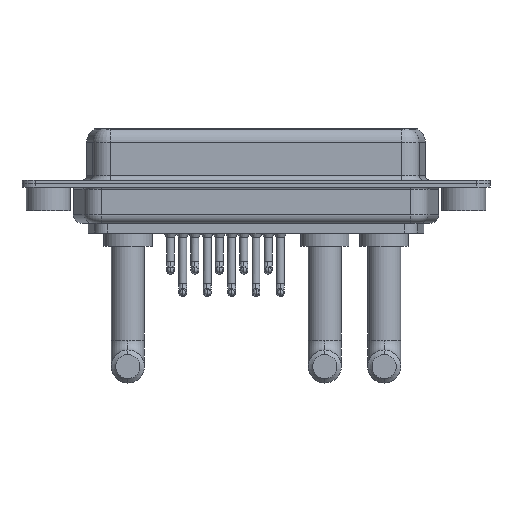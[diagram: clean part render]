
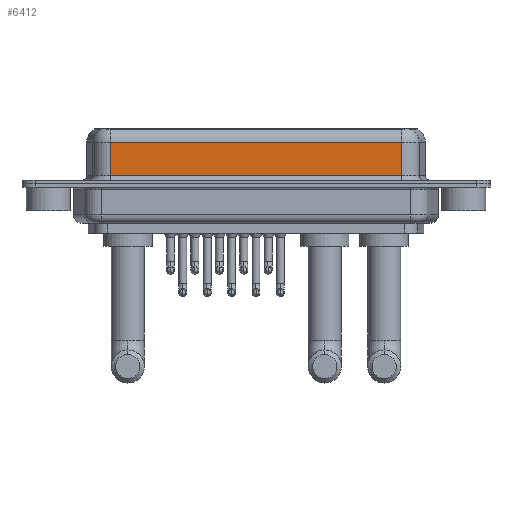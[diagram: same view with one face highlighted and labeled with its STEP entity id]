
A CAD part, front view. The second image highlights one B-rep face of the part: STEP entity #6412.
In plain terms, the highlighted planar face has unit normal (0, -1, 0).
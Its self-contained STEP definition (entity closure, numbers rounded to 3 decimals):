
#167 = CARTESIAN_POINT ( 'NONE',  ( 7.013, -3.95, 0.9 ) ) ;
#1399 = CARTESIAN_POINT ( 'NONE',  ( 40.037, -3.95, 4.65 ) ) ;
#1458 = CARTESIAN_POINT ( 'NONE',  ( 40.037, -3.95, 0.9 ) ) ;
#1975 = AXIS2_PLACEMENT_3D ( 'NONE', #12517, #11176, #11276 ) ;
#2975 = VECTOR ( 'NONE', #13521, 1000. ) ;
#3056 = VECTOR ( 'NONE', #12246, 1000. ) ;
#4353 = CARTESIAN_POINT ( 'NONE',  ( 7.013, -3.95, 6.4 ) ) ;
#5271 = VECTOR ( 'NONE', #11864, 1000. ) ;
#5887 = LINE ( 'NONE', #4353, #5271 ) ;
#6412 = ADVANCED_FACE ( 'NONE', ( #6461 ), #15302, .F. ) ;
#6461 = FACE_OUTER_BOUND ( 'NONE', #9203, .T. ) ;
#7152 = VERTEX_POINT ( 'NONE', #1399 ) ;
#7917 = ORIENTED_EDGE ( 'NONE', *, *, #9746, .T. ) ;
#8145 = LINE ( 'NONE', #16818, #17758 ) ;
#8759 = ORIENTED_EDGE ( 'NONE', *, *, #16639, .T. ) ;
#8780 = VERTEX_POINT ( 'NONE', #8987 ) ;
#8987 = CARTESIAN_POINT ( 'NONE',  ( 7.013, -3.95, 4.65 ) ) ;
#9203 = EDGE_LOOP ( 'NONE', ( #9538, #8759, #16609, #7917 ) ) ;
#9207 = EDGE_CURVE ( 'NONE', #8780, #16723, #5887, .T. ) ;
#9538 = ORIENTED_EDGE ( 'NONE', *, *, #18975, .F. ) ;
#9584 = DIRECTION ( 'NONE',  ( 0., 0., -1. ) ) ;
#9746 = EDGE_CURVE ( 'NONE', #16723, #13545, #14645, .T. ) ;
#11176 = DIRECTION ( 'NONE',  ( 0., 1., 0. ) ) ;
#11276 = DIRECTION ( 'NONE',  ( 0., 0., 1. ) ) ;
#11864 = DIRECTION ( 'NONE',  ( 0., 0., -1. ) ) ;
#12246 = DIRECTION ( 'NONE',  ( 1., 0., 0. ) ) ;
#12517 = CARTESIAN_POINT ( 'NONE',  ( 40.037, -3.95, 6.4 ) ) ;
#13153 = LINE ( 'NONE', #16323, #2975 ) ;
#13521 = DIRECTION ( 'NONE',  ( -1., 0., 0. ) ) ;
#13545 = VERTEX_POINT ( 'NONE', #16010 ) ;
#14645 = LINE ( 'NONE', #1458, #3056 ) ;
#15302 = PLANE ( 'NONE',  #1975 ) ;
#16010 = CARTESIAN_POINT ( 'NONE',  ( 40.037, -3.95, 0.9 ) ) ;
#16323 = CARTESIAN_POINT ( 'NONE',  ( 40.037, -3.95, 4.65 ) ) ;
#16609 = ORIENTED_EDGE ( 'NONE', *, *, #9207, .T. ) ;
#16639 = EDGE_CURVE ( 'NONE', #7152, #8780, #13153, .T. ) ;
#16723 = VERTEX_POINT ( 'NONE', #167 ) ;
#16818 = CARTESIAN_POINT ( 'NONE',  ( 40.037, -3.95, 6.4 ) ) ;
#17758 = VECTOR ( 'NONE', #9584, 1000. ) ;
#18975 = EDGE_CURVE ( 'NONE', #7152, #13545, #8145, .T. ) ;
